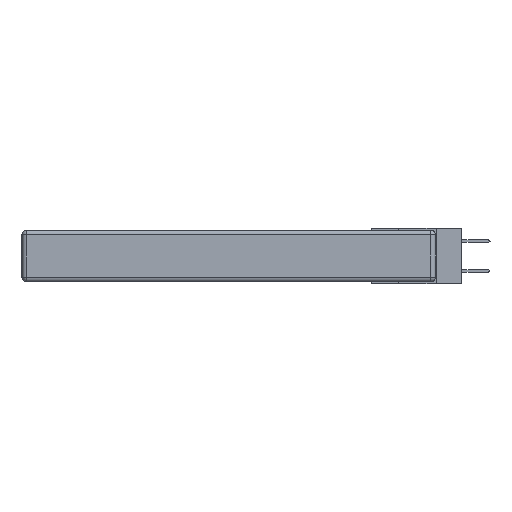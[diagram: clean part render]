
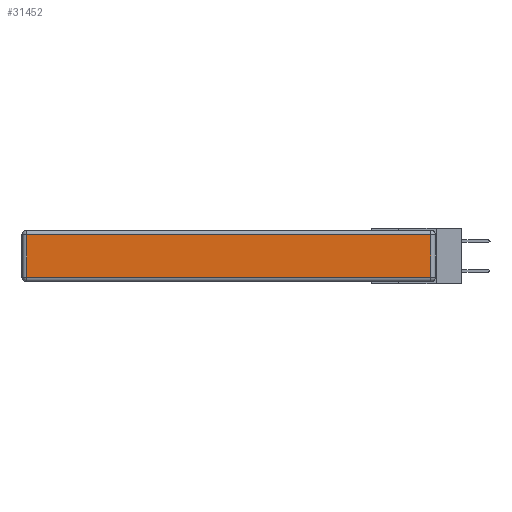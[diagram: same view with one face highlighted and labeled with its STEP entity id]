
A CAD part, left-side view. The second image highlights one B-rep face of the part: STEP entity #31452.
In plain terms, the highlighted planar face has unit normal (-1, 0, 0).
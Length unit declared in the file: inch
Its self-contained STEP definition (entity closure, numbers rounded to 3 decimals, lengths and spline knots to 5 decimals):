
#2965 = DIRECTION ( 'NONE',  ( -1., 0., 0. ) ) ;
#3234 = VECTOR ( 'NONE', #4136, 39.37008 ) ;
#4136 = DIRECTION ( 'NONE',  ( 0., 0., -1. ) ) ;
#7212 = EDGE_CURVE ( 'NONE', #20827, #24155, #28979, .T. ) ;
#8335 = DIRECTION ( 'NONE',  ( 0., -1., 0. ) ) ;
#8513 = CARTESIAN_POINT ( 'NONE',  ( 0., 2.72, -0.03 ) ) ;
#8670 = CARTESIAN_POINT ( 'NONE',  ( 0., 0., -0.313 ) ) ;
#9113 = EDGE_CURVE ( 'NONE', #24155, #9144, #27546, .T. ) ;
#9144 = VERTEX_POINT ( 'NONE', #17853 ) ;
#9749 = FACE_OUTER_BOUND ( 'NONE', #25369, .T. ) ;
#9927 = LINE ( 'NONE', #20125, #3234 ) ;
#10648 = VECTOR ( 'NONE', #29454, 39.37008 ) ;
#11105 = VECTOR ( 'NONE', #17037, 39.37008 ) ;
#11267 = ORIENTED_EDGE ( 'NONE', *, *, #9113, .T. ) ;
#13064 = CARTESIAN_POINT ( 'NONE',  ( 0., 2.75, -0.03 ) ) ;
#17037 = DIRECTION ( 'NONE',  ( 0., 0., 1. ) ) ;
#17853 = CARTESIAN_POINT ( 'NONE',  ( 0., 0.03, -0.03 ) ) ;
#18132 = PLANE ( 'NONE',  #19338 ) ;
#19338 = AXIS2_PLACEMENT_3D ( 'NONE', #23529, #2965, #29810 ) ;
#19489 = CARTESIAN_POINT ( 'NONE',  ( 0., 0.03, -0.313 ) ) ;
#19678 = VECTOR ( 'NONE', #8335, 39.37008 ) ;
#19716 = CARTESIAN_POINT ( 'NONE',  ( 0., 2.72, -0.313 ) ) ;
#20125 = CARTESIAN_POINT ( 'NONE',  ( 0., 2.72, -0.343 ) ) ;
#20827 = VERTEX_POINT ( 'NONE', #19716 ) ;
#22241 = VERTEX_POINT ( 'NONE', #8513 ) ;
#23529 = CARTESIAN_POINT ( 'NONE',  ( 0., 0., -0.343 ) ) ;
#24155 = VERTEX_POINT ( 'NONE', #19489 ) ;
#24388 = ORIENTED_EDGE ( 'NONE', *, *, #28291, .T. ) ;
#25369 = EDGE_LOOP ( 'NONE', ( #29397, #11267, #24388, #30086 ) ) ;
#26098 = EDGE_CURVE ( 'NONE', #22241, #20827, #9927, .T. ) ;
#27546 = LINE ( 'NONE', #33284, #11105 ) ;
#28291 = EDGE_CURVE ( 'NONE', #9144, #22241, #30067, .T. ) ;
#28979 = LINE ( 'NONE', #8670, #19678 ) ;
#29397 = ORIENTED_EDGE ( 'NONE', *, *, #7212, .T. ) ;
#29454 = DIRECTION ( 'NONE',  ( 0., 1., 0. ) ) ;
#29810 = DIRECTION ( 'NONE',  ( 0., 0., 1. ) ) ;
#30067 = LINE ( 'NONE', #13064, #10648 ) ;
#30086 = ORIENTED_EDGE ( 'NONE', *, *, #26098, .T. ) ;
#31452 = ADVANCED_FACE ( 'NONE', ( #9749 ), #18132, .T. ) ;
#33284 = CARTESIAN_POINT ( 'NONE',  ( 0., 0.03, -0.343 ) ) ;
